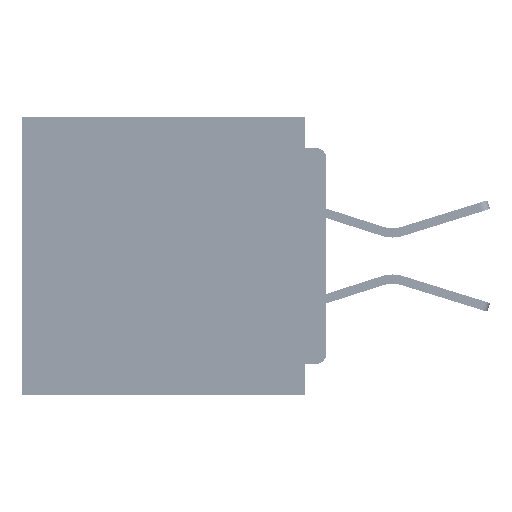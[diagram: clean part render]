
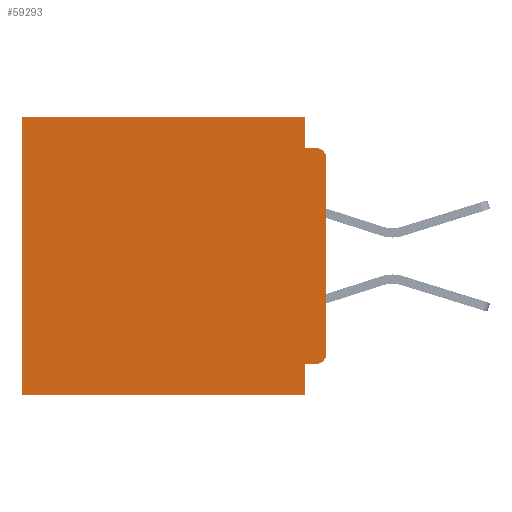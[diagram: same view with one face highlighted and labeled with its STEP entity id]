
A CAD part, left-side view. The second image highlights one B-rep face of the part: STEP entity #59293.
In plain terms, the highlighted planar face has unit normal (-1, 0, 0).
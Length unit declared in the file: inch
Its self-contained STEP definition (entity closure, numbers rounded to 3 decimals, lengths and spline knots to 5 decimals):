
#37 = CARTESIAN_POINT ( 'NONE',  ( 0.3, 0.015, -0.06 ) ) ;
#132 = VECTOR ( 'NONE', #58211, 39.37008 ) ;
#2036 = CARTESIAN_POINT ( 'NONE',  ( 0.3, 0.437, -0.4 ) ) ;
#2088 = LINE ( 'NONE', #18921, #38134 ) ;
#3489 = CARTESIAN_POINT ( 'NONE',  ( 0.3, 0., -0.34 ) ) ;
#3910 = AXIS2_PLACEMENT_3D ( 'NONE', #37, #34329, #4958 ) ;
#4207 = CARTESIAN_POINT ( 'NONE',  ( 0.3, 0.031, -0.045 ) ) ;
#4282 = CARTESIAN_POINT ( 'NONE',  ( 0.3, 0., 0. ) ) ;
#4463 = VERTEX_POINT ( 'NONE', #16892 ) ;
#4930 = EDGE_CURVE ( 'NONE', #52578, #44965, #49608, .T. ) ;
#4958 = DIRECTION ( 'NONE',  ( 0., 0., -1. ) ) ;
#5502 = CARTESIAN_POINT ( 'NONE',  ( 0.3, 0., -0.4 ) ) ;
#6081 = LINE ( 'NONE', #60806, #45254 ) ;
#7606 = EDGE_CURVE ( 'NONE', #27438, #32555, #39230, .T. ) ;
#9101 = CARTESIAN_POINT ( 'NONE',  ( 0.3, 0.437, 0. ) ) ;
#10838 = DIRECTION ( 'NONE',  ( -1., 0., 0. ) ) ;
#13126 = FACE_OUTER_BOUND ( 'NONE', #59402, .T. ) ;
#14685 = CARTESIAN_POINT ( 'NONE',  ( 0.3, 0., -0.4 ) ) ;
#16543 = PLANE ( 'NONE',  #24033 ) ;
#16560 = EDGE_CURVE ( 'NONE', #24430, #4463, #49735, .T. ) ;
#16579 = ORIENTED_EDGE ( 'NONE', *, *, #22206, .F. ) ;
#16892 = CARTESIAN_POINT ( 'NONE',  ( 0.3, 0.031, -0.4 ) ) ;
#17002 = EDGE_CURVE ( 'NONE', #52578, #24430, #2088, .T. ) ;
#18921 = CARTESIAN_POINT ( 'NONE',  ( 0.3, 0., -0.355 ) ) ;
#19455 = ORIENTED_EDGE ( 'NONE', *, *, #16560, .F. ) ;
#22206 = EDGE_CURVE ( 'NONE', #51690, #44965, #38985, .T. ) ;
#22509 = CIRCLE ( 'NONE', #3910, 0.015 ) ;
#23979 = CARTESIAN_POINT ( 'NONE',  ( 0.3, 0.031, 0. ) ) ;
#24033 = AXIS2_PLACEMENT_3D ( 'NONE', #55902, #26327, #60793 ) ;
#24430 = VERTEX_POINT ( 'NONE', #28085 ) ;
#24544 = CARTESIAN_POINT ( 'NONE',  ( 0.3, 0.015, -0.045 ) ) ;
#24924 = EDGE_CURVE ( 'NONE', #55493, #58393, #56436, .T. ) ;
#25556 = DIRECTION ( 'NONE',  ( 0., 0., -1. ) ) ;
#26327 = DIRECTION ( 'NONE',  ( 1., 0., 0. ) ) ;
#26335 = DIRECTION ( 'NONE',  ( 0., 0., -1. ) ) ;
#27396 = VECTOR ( 'NONE', #53814, 39.37008 ) ;
#27397 = LINE ( 'NONE', #5502, #62086 ) ;
#27438 = VERTEX_POINT ( 'NONE', #9101 ) ;
#28085 = CARTESIAN_POINT ( 'NONE',  ( 0.3, 0.031, -0.355 ) ) ;
#28494 = CARTESIAN_POINT ( 'NONE',  ( 0.3, 0.015, -0.355 ) ) ;
#28622 = VECTOR ( 'NONE', #38569, 39.37008 ) ;
#28649 = CARTESIAN_POINT ( 'NONE',  ( 0.3, 0.437, -0.4 ) ) ;
#29225 = ORIENTED_EDGE ( 'NONE', *, *, #57736, .T. ) ;
#31430 = CARTESIAN_POINT ( 'NONE',  ( 0.3, 0., -0.06 ) ) ;
#32555 = VERTEX_POINT ( 'NONE', #2036 ) ;
#34329 = DIRECTION ( 'NONE',  ( -1., 0., 0. ) ) ;
#34936 = ORIENTED_EDGE ( 'NONE', *, *, #49286, .F. ) ;
#37686 = DIRECTION ( 'NONE',  ( 0., -1., 0. ) ) ;
#38134 = VECTOR ( 'NONE', #48366, 39.37008 ) ;
#38569 = DIRECTION ( 'NONE',  ( 0., 1., 0. ) ) ;
#38645 = LINE ( 'NONE', #4282, #28622 ) ;
#38985 = LINE ( 'NONE', #14685, #27396 ) ;
#39230 = LINE ( 'NONE', #28649, #132 ) ;
#40231 = CARTESIAN_POINT ( 'NONE',  ( 0.3, 0.015, -0.34 ) ) ;
#44846 = VECTOR ( 'NONE', #37686, 39.37008 ) ;
#44965 = VERTEX_POINT ( 'NONE', #3489 ) ;
#45184 = DIRECTION ( 'NONE',  ( 0., 0., -1. ) ) ;
#45254 = VECTOR ( 'NONE', #26335, 39.37008 ) ;
#45502 = ORIENTED_EDGE ( 'NONE', *, *, #54805, .T. ) ;
#46588 = ORIENTED_EDGE ( 'NONE', *, *, #17002, .F. ) ;
#47833 = CARTESIAN_POINT ( 'NONE',  ( 0.3, 0., -0.045 ) ) ;
#48366 = DIRECTION ( 'NONE',  ( 0., 1., 0. ) ) ;
#49286 = EDGE_CURVE ( 'NONE', #54347, #55493, #6081, .T. ) ;
#49608 = CIRCLE ( 'NONE', #50926, 0.015 ) ;
#49704 = DIRECTION ( 'NONE',  ( 0., 1., 0. ) ) ;
#49735 = LINE ( 'NONE', #50108, #61293 ) ;
#50108 = CARTESIAN_POINT ( 'NONE',  ( 0.3, 0.031, -0.4 ) ) ;
#50691 = ORIENTED_EDGE ( 'NONE', *, *, #7606, .T. ) ;
#50926 = AXIS2_PLACEMENT_3D ( 'NONE', #40231, #10838, #45184 ) ;
#51690 = VERTEX_POINT ( 'NONE', #31430 ) ;
#52578 = VERTEX_POINT ( 'NONE', #28494 ) ;
#53814 = DIRECTION ( 'NONE',  ( 0., 0., -1. ) ) ;
#54347 = VERTEX_POINT ( 'NONE', #23979 ) ;
#54805 = EDGE_CURVE ( 'NONE', #54347, #27438, #38645, .T. ) ;
#55493 = VERTEX_POINT ( 'NONE', #4207 ) ;
#55902 = CARTESIAN_POINT ( 'NONE',  ( 0.3, 0., -0.4 ) ) ;
#56436 = LINE ( 'NONE', #47833, #44846 ) ;
#57736 = EDGE_CURVE ( 'NONE', #51690, #58393, #22509, .T. ) ;
#58211 = DIRECTION ( 'NONE',  ( 0., 0., -1. ) ) ;
#58393 = VERTEX_POINT ( 'NONE', #24544 ) ;
#59293 = ADVANCED_FACE ( 'NONE', ( #13126 ), #16543, .F. ) ;
#59402 = EDGE_LOOP ( 'NONE', ( #16579, #29225, #61039, #34936, #45502, #50691, #62198, #19455, #46588, #60564 ) ) ;
#60564 = ORIENTED_EDGE ( 'NONE', *, *, #4930, .T. ) ;
#60793 = DIRECTION ( 'NONE',  ( 0., 0., -1. ) ) ;
#60806 = CARTESIAN_POINT ( 'NONE',  ( 0.3, 0.031, 0. ) ) ;
#61039 = ORIENTED_EDGE ( 'NONE', *, *, #24924, .F. ) ;
#61293 = VECTOR ( 'NONE', #25556, 39.37008 ) ;
#61715 = EDGE_CURVE ( 'NONE', #4463, #32555, #27397, .T. ) ;
#62086 = VECTOR ( 'NONE', #49704, 39.37008 ) ;
#62198 = ORIENTED_EDGE ( 'NONE', *, *, #61715, .F. ) ;
